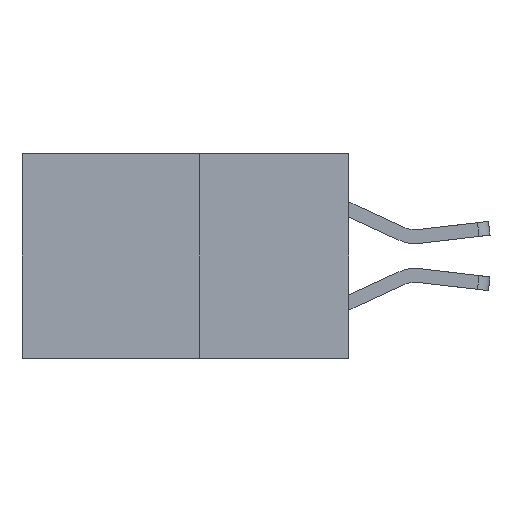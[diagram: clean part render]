
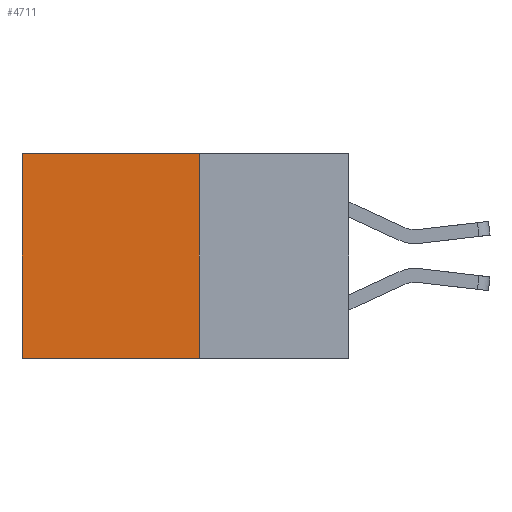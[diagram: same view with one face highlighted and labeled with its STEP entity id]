
A CAD part, left-side view. The second image highlights one B-rep face of the part: STEP entity #4711.
In plain terms, the highlighted planar face has unit normal (-1, 0, 0).
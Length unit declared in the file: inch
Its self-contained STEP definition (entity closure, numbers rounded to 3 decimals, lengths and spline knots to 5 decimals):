
#284 = CARTESIAN_POINT ( 'NONE',  ( 0.277, 0.27, 0. ) ) ;
#769 = LINE ( 'NONE', #5096, #6883 ) ;
#852 = EDGE_CURVE ( 'NONE', #2387, #2214, #2367, .T. ) ;
#1016 = FACE_OUTER_BOUND ( 'NONE', #6814, .T. ) ;
#1258 = LINE ( 'NONE', #4791, #7311 ) ;
#1429 = AXIS2_PLACEMENT_3D ( 'NONE', #5801, #5458, #5412 ) ;
#2214 = VERTEX_POINT ( 'NONE', #2678 ) ;
#2367 = LINE ( 'NONE', #9522, #5744 ) ;
#2378 = ORIENTED_EDGE ( 'NONE', *, *, #5637, .F. ) ;
#2387 = VERTEX_POINT ( 'NONE', #5779 ) ;
#2678 = CARTESIAN_POINT ( 'NONE',  ( 0.277, 0.59, -0.37 ) ) ;
#3127 = VERTEX_POINT ( 'NONE', #4919 ) ;
#3414 = LINE ( 'NONE', #6549, #5482 ) ;
#3981 = EDGE_CURVE ( 'NONE', #9449, #2387, #3414, .T. ) ;
#3991 = DIRECTION ( 'NONE',  ( 0., 0., -1. ) ) ;
#4711 = ADVANCED_FACE ( 'NONE', ( #1016 ), #5471, .F. ) ;
#4730 = EDGE_CURVE ( 'NONE', #3127, #2214, #769, .T. ) ;
#4791 = CARTESIAN_POINT ( 'NONE',  ( 0.277, 0.27, -0.37 ) ) ;
#4802 = DIRECTION ( 'NONE',  ( 0., 0., -1. ) ) ;
#4919 = CARTESIAN_POINT ( 'NONE',  ( 0.277, 0.27, -0.37 ) ) ;
#5096 = CARTESIAN_POINT ( 'NONE',  ( 0.277, 0.27, -0.37 ) ) ;
#5335 = DIRECTION ( 'NONE',  ( 0., 1., 0. ) ) ;
#5412 = DIRECTION ( 'NONE',  ( 0., 0., -1. ) ) ;
#5458 = DIRECTION ( 'NONE',  ( 1., 0., 0. ) ) ;
#5471 = PLANE ( 'NONE',  #1429 ) ;
#5482 = VECTOR ( 'NONE', #6560, 39.37008 ) ;
#5637 = EDGE_CURVE ( 'NONE', #9449, #3127, #1258, .T. ) ;
#5744 = VECTOR ( 'NONE', #3991, 39.37008 ) ;
#5779 = CARTESIAN_POINT ( 'NONE',  ( 0.277, 0.59, 0. ) ) ;
#5801 = CARTESIAN_POINT ( 'NONE',  ( 0.277, 0.27, -0.37 ) ) ;
#6549 = CARTESIAN_POINT ( 'NONE',  ( 0.277, 0.27, 0. ) ) ;
#6560 = DIRECTION ( 'NONE',  ( 0., 1., 0. ) ) ;
#6742 = ORIENTED_EDGE ( 'NONE', *, *, #852, .T. ) ;
#6814 = EDGE_LOOP ( 'NONE', ( #6742, #9674, #2378, #6996 ) ) ;
#6883 = VECTOR ( 'NONE', #5335, 39.37008 ) ;
#6996 = ORIENTED_EDGE ( 'NONE', *, *, #3981, .T. ) ;
#7311 = VECTOR ( 'NONE', #4802, 39.37008 ) ;
#9449 = VERTEX_POINT ( 'NONE', #284 ) ;
#9522 = CARTESIAN_POINT ( 'NONE',  ( 0.277, 0.59, -0.37 ) ) ;
#9674 = ORIENTED_EDGE ( 'NONE', *, *, #4730, .F. ) ;
